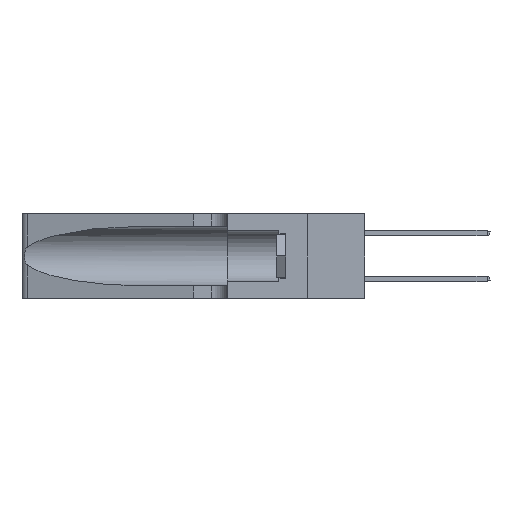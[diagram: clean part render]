
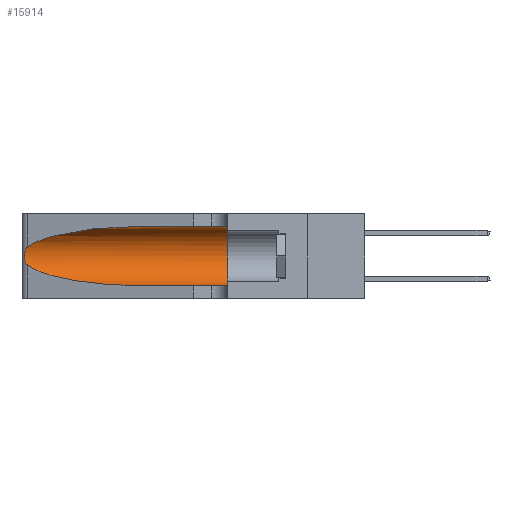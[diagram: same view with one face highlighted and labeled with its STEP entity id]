
A CAD part, left-side view. The second image highlights one B-rep face of the part: STEP entity #15914.
In plain terms, the highlighted cylindrical face has radius 3.308 mm (diameter 6.617 mm), a partial arc.
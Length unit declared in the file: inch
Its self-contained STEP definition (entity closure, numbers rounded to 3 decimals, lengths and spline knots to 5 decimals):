
#713 = CARTESIAN_POINT ( 'NONE',  ( 0.1305, 0.35, 0.31525 ) ) ;
#1256 = CARTESIAN_POINT ( 'NONE',  ( 0.25555, 1.22994, 0.2215 ) ) ;
#1392 = CARTESIAN_POINT ( 'NONE',  ( 0.25487, 1.22718, 0.14631 ) ) ;
#2409 = DIRECTION ( 'NONE',  ( 0., -1., 0. ) ) ;
#2824 = CARTESIAN_POINT ( 'NONE',  ( 0.18966, 0.96281, 0.31525 ) ) ;
#3806 = DIRECTION ( 'NONE',  ( 0., -1., 0. ) ) ;
#4248 = CARTESIAN_POINT ( 'NONE',  ( 0.25639, 1.23184, 0.21858 ) ) ;
#4361 =( BOUNDED_CURVE ( )  B_SPLINE_CURVE ( 3, ( #38244, #17582, #32370, #5684 ),
 .UNSPECIFIED., .F., .F. ) 
 B_SPLINE_CURVE_WITH_KNOTS ( ( 4, 4 ),
 ( 3.44316, 4.71239 ),
 .UNSPECIFIED. ) 
 CURVE ( )  GEOMETRIC_REPRESENTATION_ITEM ( )  RATIONAL_B_SPLINE_CURVE ( ( 1., 0.87, 0.87, 1. ) ) 
 REPRESENTATION_ITEM ( '' )  );
#4629 = VERTEX_POINT ( 'NONE', #713 ) ;
#5007 = ORIENTED_EDGE ( 'NONE', *, *, #31080, .T. ) ;
#5217 = DIRECTION ( 'NONE',  ( 0., 1., 0. ) ) ;
#5684 = CARTESIAN_POINT ( 'NONE',  ( 0.1305, 0.72297, 0.05475 ) ) ;
#5809 = CARTESIAN_POINT ( 'NONE',  ( 0.1305, 0.72297, 0.05475 ) ) ;
#7188 = CARTESIAN_POINT ( 'NONE',  ( 0.25854, 1.2359, 0.20912 ) ) ;
#8334 = LINE ( 'NONE', #24619, #30241 ) ;
#8348 = DIRECTION ( 'NONE',  ( 0., 0., -1. ) ) ;
#8774 = CARTESIAN_POINT ( 'NONE',  ( 0.2373, 1.15595, 0.28018 ) ) ;
#9219 = AXIS2_PLACEMENT_3D ( 'NONE', #23064, #5217, #26060 ) ;
#10194 = CARTESIAN_POINT ( 'NONE',  ( 0.26075, 1.23896, 0.19203 ) ) ;
#10711 = EDGE_CURVE ( 'NONE', #12674, #4629, #8334, .T. ) ;
#11136 = VECTOR ( 'NONE', #33248, 39.37008 ) ;
#11151 = ORIENTED_EDGE ( 'NONE', *, *, #30678, .T. ) ;
#11353 = CARTESIAN_POINT ( 'NONE',  ( 0.1305, 1.61858, 0.185 ) ) ;
#12428 = EDGE_CURVE ( 'NONE', #4629, #37618, #21928, .T. ) ;
#12674 = VERTEX_POINT ( 'NONE', #29930 ) ;
#13137 = EDGE_CURVE ( 'NONE', #22584, #13167, #4361, .T. ) ;
#13167 = VERTEX_POINT ( 'NONE', #5809 ) ;
#13235 = CARTESIAN_POINT ( 'NONE',  ( 0.26017, 1.23833, 0.17102 ) ) ;
#14033 = ORIENTED_EDGE ( 'NONE', *, *, #12428, .F. ) ;
#15914 = ADVANCED_FACE ( 'NONE', ( #22628 ), #37423, .F. ) ;
#16277 = CARTESIAN_POINT ( 'NONE',  ( 0.25789, 1.23486, 0.15765 ) ) ;
#17480 = EDGE_LOOP ( 'NONE', ( #5007, #22735, #19524, #11151, #14033, #29835 ) ) ;
#17582 = CARTESIAN_POINT ( 'NONE',  ( 0.2373, 1.15595, 0.08982 ) ) ;
#18173 = LINE ( 'NONE', #27443, #11136 ) ;
#18881 = CARTESIAN_POINT ( 'NONE',  ( 0.25487, 1.22718, 0.14631 ) ) ;
#19229 = VERTEX_POINT ( 'NONE', #23038 ) ;
#19241 = CARTESIAN_POINT ( 'NONE',  ( 0.25555, 1.22993, 0.14849 ) ) ;
#19524 = ORIENTED_EDGE ( 'NONE', *, *, #13137, .T. ) ;
#21928 = CIRCLE ( 'NONE', #9219, 0.13025 ) ;
#22584 = VERTEX_POINT ( 'NONE', #18881 ) ;
#22628 = FACE_OUTER_BOUND ( 'NONE', #17480, .T. ) ;
#22735 = ORIENTED_EDGE ( 'NONE', *, *, #33390, .T. ) ;
#23038 = CARTESIAN_POINT ( 'NONE',  ( 0.25487, 1.22718, 0.22369 ) ) ;
#23064 = CARTESIAN_POINT ( 'NONE',  ( 0.1305, 0.35, 0.185 ) ) ;
#23632 = CARTESIAN_POINT ( 'NONE',  ( 0.1305, 0.72297, 0.31525 ) ) ;
#23834 = CARTESIAN_POINT ( 'NONE',  ( 0.1305, 0.35, 0.05475 ) ) ;
#24619 = CARTESIAN_POINT ( 'NONE',  ( 0.1305, 1.61858, 0.31525 ) ) ;
#25084 = CARTESIAN_POINT ( 'NONE',  ( 0.25787, 1.23484, 0.2124 ) ) ;
#26060 = DIRECTION ( 'NONE',  ( 0., 0., 1. ) ) ;
#27443 = CARTESIAN_POINT ( 'NONE',  ( 0.1305, 1.61858, 0.05475 ) ) ;
#28071 = CARTESIAN_POINT ( 'NONE',  ( 0.26018, 1.23835, 0.19895 ) ) ;
#29603 = CARTESIAN_POINT ( 'NONE',  ( 0.25487, 1.22718, 0.22369 ) ) ;
#29835 = ORIENTED_EDGE ( 'NONE', *, *, #10711, .F. ) ;
#29930 = CARTESIAN_POINT ( 'NONE',  ( 0.1305, 0.72297, 0.31525 ) ) ;
#30241 = VECTOR ( 'NONE', #3806, 39.37008 ) ;
#30678 = EDGE_CURVE ( 'NONE', #13167, #37618, #18173, .T. ) ;
#30762 =( BOUNDED_CURVE ( )  B_SPLINE_CURVE ( 3, ( #23632, #2824, #8774, #29603 ),
 .UNSPECIFIED., .F., .F. ) 
 B_SPLINE_CURVE_WITH_KNOTS ( ( 4, 4 ),
 ( 1.5708, 2.84003 ),
 .UNSPECIFIED. ) 
 CURVE ( )  GEOMETRIC_REPRESENTATION_ITEM ( )  RATIONAL_B_SPLINE_CURVE ( ( 1., 0.87, 0.87, 1. ) ) 
 REPRESENTATION_ITEM ( '' )  );
#31035 = CARTESIAN_POINT ( 'NONE',  ( 0.26075, 1.23896, 0.178 ) ) ;
#31080 = EDGE_CURVE ( 'NONE', #12674, #19229, #30762, .T. ) ;
#32370 = CARTESIAN_POINT ( 'NONE',  ( 0.18966, 0.96281, 0.05475 ) ) ;
#33248 = DIRECTION ( 'NONE',  ( 0., -1., 0. ) ) ;
#33390 = EDGE_CURVE ( 'NONE', #19229, #22584, #35264, .T. ) ;
#34019 = CARTESIAN_POINT ( 'NONE',  ( 0.25856, 1.23593, 0.16098 ) ) ;
#35264 = B_SPLINE_CURVE_WITH_KNOTS ( 'NONE', 3,
 ( #36833, #1256, #4248, #25084, #7188, #28071, #10194, #31035, #13235, #34019, #16277, #36959, #19241, #1392 ),
 .UNSPECIFIED., .F., .F.,
 ( 4, 2, 2, 2, 2, 2, 4 ),
 ( 0., 0.00027, 0.00053, 0.00107, 0.0016, 0.00187, 0.00214 ),
 .UNSPECIFIED. ) ;
#36833 = CARTESIAN_POINT ( 'NONE',  ( 0.25487, 1.22718, 0.22369 ) ) ;
#36959 = CARTESIAN_POINT ( 'NONE',  ( 0.25639, 1.23186, 0.15144 ) ) ;
#37423 = CYLINDRICAL_SURFACE ( 'NONE', #37566, 0.13025 ) ;
#37566 = AXIS2_PLACEMENT_3D ( 'NONE', #11353, #2409, #8348 ) ;
#37618 = VERTEX_POINT ( 'NONE', #23834 ) ;
#38244 = CARTESIAN_POINT ( 'NONE',  ( 0.25487, 1.22718, 0.14631 ) ) ;
